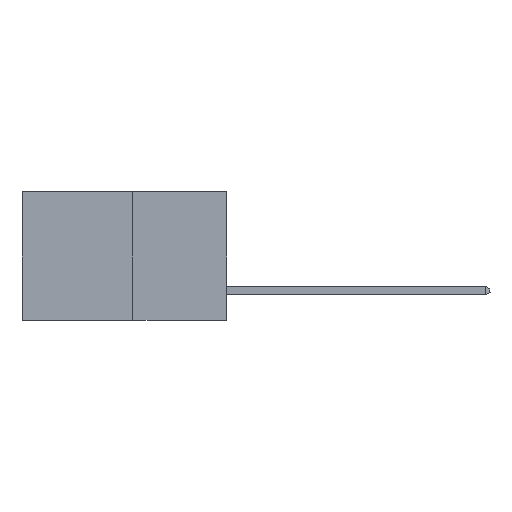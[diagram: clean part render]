
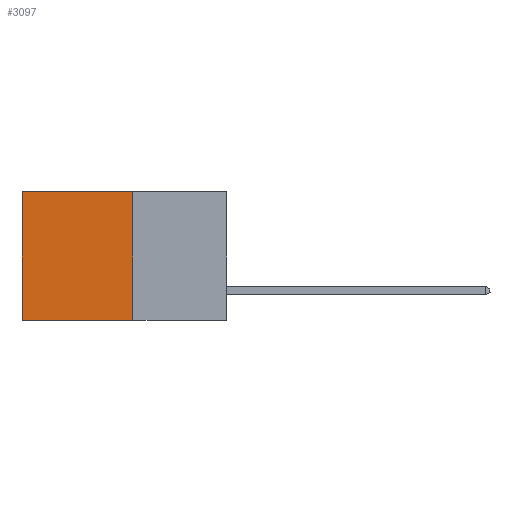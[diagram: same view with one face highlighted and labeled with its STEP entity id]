
A CAD part, left-side view. The second image highlights one B-rep face of the part: STEP entity #3097.
In plain terms, the highlighted planar face has unit normal (-1, 0, 0).
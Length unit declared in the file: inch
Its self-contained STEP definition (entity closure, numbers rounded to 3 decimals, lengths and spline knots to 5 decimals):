
#210 = FACE_OUTER_BOUND ( 'NONE', #10974, .T. ) ;
#945 = CARTESIAN_POINT ( 'NONE',  ( 0.277, 0.59, -0.37 ) ) ;
#2362 = CARTESIAN_POINT ( 'NONE',  ( 0.277, 0.27, -0.37 ) ) ;
#2930 = ORIENTED_EDGE ( 'NONE', *, *, #20058, .T. ) ;
#3097 = ADVANCED_FACE ( 'NONE', ( #210 ), #7318, .F. ) ;
#3376 = VECTOR ( 'NONE', #21940, 39.37008 ) ;
#4273 = VERTEX_POINT ( 'NONE', #18190 ) ;
#4637 = VECTOR ( 'NONE', #19273, 39.37008 ) ;
#5458 = CARTESIAN_POINT ( 'NONE',  ( 0.277, 0.27, -0.37 ) ) ;
#6957 = DIRECTION ( 'NONE',  ( 0., 0., -1. ) ) ;
#7078 = DIRECTION ( 'NONE',  ( 1., 0., 0. ) ) ;
#7239 = CARTESIAN_POINT ( 'NONE',  ( 0.277, 0.27, -0.37 ) ) ;
#7318 = PLANE ( 'NONE',  #9836 ) ;
#7759 = ORIENTED_EDGE ( 'NONE', *, *, #9964, .F. ) ;
#8175 = CARTESIAN_POINT ( 'NONE',  ( 0.277, 0.27, 0. ) ) ;
#9080 = LINE ( 'NONE', #2362, #22604 ) ;
#9757 = EDGE_CURVE ( 'NONE', #4273, #13403, #13685, .T. ) ;
#9836 = AXIS2_PLACEMENT_3D ( 'NONE', #7239, #7078, #6957 ) ;
#9964 = EDGE_CURVE ( 'NONE', #15828, #4273, #9080, .T. ) ;
#10974 = EDGE_LOOP ( 'NONE', ( #20036, #18932, #7759, #2930 ) ) ;
#11856 = CARTESIAN_POINT ( 'NONE',  ( 0.277, 0.59, 0. ) ) ;
#13290 = CARTESIAN_POINT ( 'NONE',  ( 0.277, 0.27, 0. ) ) ;
#13349 = VERTEX_POINT ( 'NONE', #11856 ) ;
#13403 = VERTEX_POINT ( 'NONE', #21205 ) ;
#13685 = LINE ( 'NONE', #5458, #3376 ) ;
#14400 = LINE ( 'NONE', #8175, #4637 ) ;
#15828 = VERTEX_POINT ( 'NONE', #13290 ) ;
#16895 = LINE ( 'NONE', #945, #21800 ) ;
#17451 = DIRECTION ( 'NONE',  ( 0., 0., -1. ) ) ;
#18190 = CARTESIAN_POINT ( 'NONE',  ( 0.277, 0.27, -0.37 ) ) ;
#18887 = DIRECTION ( 'NONE',  ( 0., 0., -1. ) ) ;
#18932 = ORIENTED_EDGE ( 'NONE', *, *, #9757, .F. ) ;
#19273 = DIRECTION ( 'NONE',  ( 0., 1., 0. ) ) ;
#20036 = ORIENTED_EDGE ( 'NONE', *, *, #21436, .T. ) ;
#20058 = EDGE_CURVE ( 'NONE', #15828, #13349, #14400, .T. ) ;
#21205 = CARTESIAN_POINT ( 'NONE',  ( 0.277, 0.59, -0.37 ) ) ;
#21436 = EDGE_CURVE ( 'NONE', #13349, #13403, #16895, .T. ) ;
#21800 = VECTOR ( 'NONE', #17451, 39.37008 ) ;
#21940 = DIRECTION ( 'NONE',  ( 0., 1., 0. ) ) ;
#22604 = VECTOR ( 'NONE', #18887, 39.37008 ) ;
